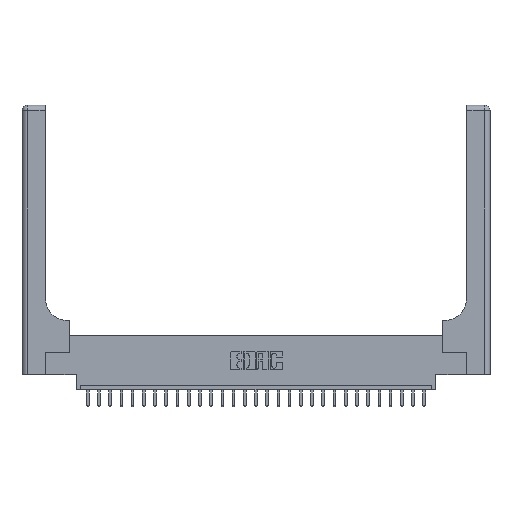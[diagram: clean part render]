
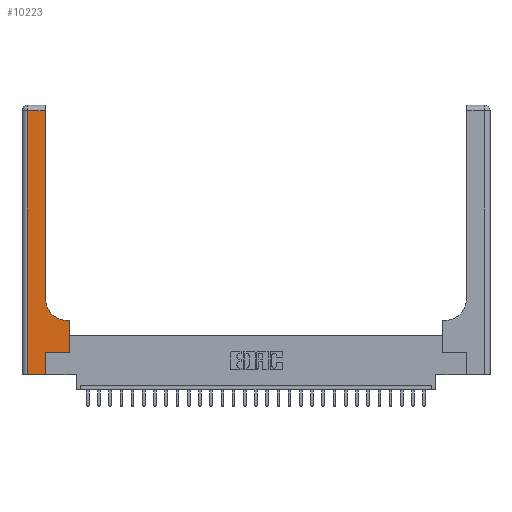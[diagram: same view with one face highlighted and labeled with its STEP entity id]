
A CAD part, top view. The second image highlights one B-rep face of the part: STEP entity #10223.
In plain terms, the highlighted planar face has unit normal (0, 0, 1).
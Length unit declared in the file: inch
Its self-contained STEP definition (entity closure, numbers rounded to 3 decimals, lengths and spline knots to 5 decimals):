
#184 = CARTESIAN_POINT ( 'NONE',  ( 0.06, 2.94, 0.37 ) ) ;
#251 = EDGE_CURVE ( 'NONE', #1539, #9249, #9373, .T. ) ;
#793 = DIRECTION ( 'NONE',  ( -1., 0., 0. ) ) ;
#899 = VECTOR ( 'NONE', #25595, 39.37008 ) ;
#934 = DIRECTION ( 'NONE',  ( 0., 0., -1. ) ) ;
#1321 = ORIENTED_EDGE ( 'NONE', *, *, #22960, .T. ) ;
#1361 = CARTESIAN_POINT ( 'NONE',  ( 0., 2.94, 0.37 ) ) ;
#1539 = VERTEX_POINT ( 'NONE', #25438 ) ;
#1732 = VECTOR ( 'NONE', #4693, 39.37008 ) ;
#2253 = DIRECTION ( 'NONE',  ( 1., 0., 0. ) ) ;
#2296 = DIRECTION ( 'NONE',  ( 1., 0., 0. ) ) ;
#2691 = CARTESIAN_POINT ( 'NONE',  ( 0.528, 0.6, 0.37 ) ) ;
#2806 = EDGE_CURVE ( 'NONE', #9249, #11494, #14113, .T. ) ;
#2842 = CARTESIAN_POINT ( 'NONE',  ( 0.528, 0.25, 0.37 ) ) ;
#2892 = EDGE_CURVE ( 'NONE', #25026, #9615, #23843, .T. ) ;
#3754 = ORIENTED_EDGE ( 'NONE', *, *, #17704, .T. ) ;
#3847 = CARTESIAN_POINT ( 'NONE',  ( 0.265, 0.25, 0.37 ) ) ;
#4004 = VECTOR ( 'NONE', #11641, 39.37008 ) ;
#4065 = ORIENTED_EDGE ( 'NONE', *, *, #2892, .T. ) ;
#4419 = VECTOR ( 'NONE', #2253, 39.37008 ) ;
#4458 = EDGE_CURVE ( 'NONE', #9615, #6874, #25552, .T. ) ;
#4693 = DIRECTION ( 'NONE',  ( 0., 1., 0. ) ) ;
#4838 = CARTESIAN_POINT ( 'NONE',  ( 0.51, 0.6, 0.37 ) ) ;
#5133 = CARTESIAN_POINT ( 'NONE',  ( 0.265, 0.25, 0.37 ) ) ;
#5136 = LINE ( 'NONE', #2842, #899 ) ;
#5912 = EDGE_LOOP ( 'NONE', ( #14250, #24759, #9416, #4065, #6249, #3754, #1321, #21171, #6178 ) ) ;
#5943 = EDGE_CURVE ( 'NONE', #23409, #16867, #10422, .T. ) ;
#6072 = DIRECTION ( 'NONE',  ( 1., 0., 0. ) ) ;
#6178 = ORIENTED_EDGE ( 'NONE', *, *, #23289, .T. ) ;
#6249 = ORIENTED_EDGE ( 'NONE', *, *, #4458, .T. ) ;
#6339 = VECTOR ( 'NONE', #21381, 39.37008 ) ;
#6652 = DIRECTION ( 'NONE',  ( -1., 0., 0. ) ) ;
#6796 = AXIS2_PLACEMENT_3D ( 'NONE', #25287, #934, #793 ) ;
#6874 = VERTEX_POINT ( 'NONE', #5133 ) ;
#7224 = CARTESIAN_POINT ( 'NONE',  ( 0.265, 0., 0.37 ) ) ;
#7334 = CARTESIAN_POINT ( 'NONE',  ( 0.06, 3., 0.37 ) ) ;
#7495 = EDGE_CURVE ( 'NONE', #11494, #25026, #22037, .T. ) ;
#7765 = CIRCLE ( 'NONE', #14214, 0.25 ) ;
#8624 = FACE_OUTER_BOUND ( 'NONE', #5912, .T. ) ;
#9249 = VERTEX_POINT ( 'NONE', #13426 ) ;
#9373 = LINE ( 'NONE', #23672, #6339 ) ;
#9416 = ORIENTED_EDGE ( 'NONE', *, *, #7495, .T. ) ;
#9615 = VERTEX_POINT ( 'NONE', #16205 ) ;
#10165 = VECTOR ( 'NONE', #13708, 39.37008 ) ;
#10223 = ADVANCED_FACE ( 'NONE', ( #8624 ), #18827, .F. ) ;
#10375 = CARTESIAN_POINT ( 'NONE',  ( 0.51, 0.85, 0.37 ) ) ;
#10422 = LINE ( 'NONE', #20661, #23308 ) ;
#11494 = VERTEX_POINT ( 'NONE', #184 ) ;
#11641 = DIRECTION ( 'NONE',  ( 0., -1., 0. ) ) ;
#13426 = CARTESIAN_POINT ( 'NONE',  ( 0.26, 2.94, 0.37 ) ) ;
#13708 = DIRECTION ( 'NONE',  ( -1., 0., 0. ) ) ;
#14030 = CARTESIAN_POINT ( 'NONE',  ( 0.06, 0., 0.37 ) ) ;
#14113 = LINE ( 'NONE', #1361, #10165 ) ;
#14214 = AXIS2_PLACEMENT_3D ( 'NONE', #10375, #16570, #6072 ) ;
#14250 = ORIENTED_EDGE ( 'NONE', *, *, #251, .T. ) ;
#16205 = CARTESIAN_POINT ( 'NONE',  ( 0.265, 0., 0.37 ) ) ;
#16570 = DIRECTION ( 'NONE',  ( 0., 0., -1. ) ) ;
#16867 = VERTEX_POINT ( 'NONE', #4838 ) ;
#17704 = EDGE_CURVE ( 'NONE', #6874, #23167, #22695, .T. ) ;
#17912 = CARTESIAN_POINT ( 'NONE',  ( 0.528, 0.25, 0.37 ) ) ;
#18827 = PLANE ( 'NONE',  #6796 ) ;
#19179 = VECTOR ( 'NONE', #2296, 39.37008 ) ;
#19778 = CARTESIAN_POINT ( 'NONE',  ( 0., 0., 0.37 ) ) ;
#20661 = CARTESIAN_POINT ( 'NONE',  ( 0.26, 0.6, 0.37 ) ) ;
#21171 = ORIENTED_EDGE ( 'NONE', *, *, #5943, .T. ) ;
#21381 = DIRECTION ( 'NONE',  ( 0., 1., 0. ) ) ;
#22037 = LINE ( 'NONE', #7334, #4004 ) ;
#22695 = LINE ( 'NONE', #3847, #4419 ) ;
#22960 = EDGE_CURVE ( 'NONE', #23167, #23409, #5136, .T. ) ;
#23167 = VERTEX_POINT ( 'NONE', #17912 ) ;
#23289 = EDGE_CURVE ( 'NONE', #16867, #1539, #7765, .T. ) ;
#23308 = VECTOR ( 'NONE', #6652, 39.37008 ) ;
#23409 = VERTEX_POINT ( 'NONE', #2691 ) ;
#23672 = CARTESIAN_POINT ( 'NONE',  ( 0.26, 3., 0.37 ) ) ;
#23843 = LINE ( 'NONE', #19778, #19179 ) ;
#24759 = ORIENTED_EDGE ( 'NONE', *, *, #2806, .T. ) ;
#25026 = VERTEX_POINT ( 'NONE', #14030 ) ;
#25287 = CARTESIAN_POINT ( 'NONE',  ( 0., 3., 0.37 ) ) ;
#25438 = CARTESIAN_POINT ( 'NONE',  ( 0.26, 0.85, 0.37 ) ) ;
#25552 = LINE ( 'NONE', #7224, #1732 ) ;
#25595 = DIRECTION ( 'NONE',  ( 0., 1., 0. ) ) ;
